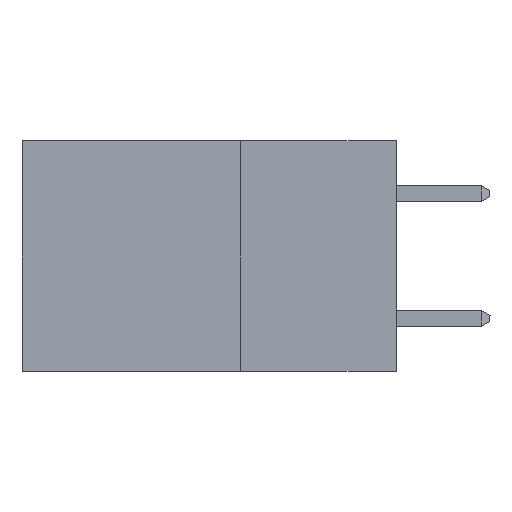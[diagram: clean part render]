
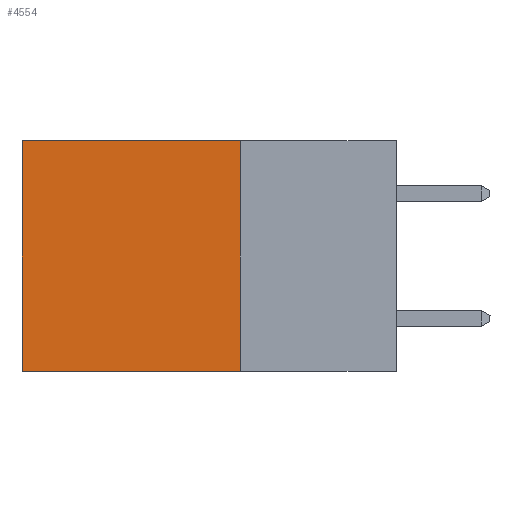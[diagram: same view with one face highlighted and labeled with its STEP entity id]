
A CAD part, left-side view. The second image highlights one B-rep face of the part: STEP entity #4554.
In plain terms, the highlighted planar face has unit normal (-1, 0, 0).
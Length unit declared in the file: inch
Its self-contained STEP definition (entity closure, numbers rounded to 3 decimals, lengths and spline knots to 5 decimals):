
#431 = EDGE_LOOP ( 'NONE', ( #10755, #3207, #16544, #15419 ) ) ;
#739 = CARTESIAN_POINT ( 'NONE',  ( 0.2615, 0.25, 0. ) ) ;
#2113 = EDGE_CURVE ( 'NONE', #11427, #13309, #3896, .T. ) ;
#2519 = LINE ( 'NONE', #15623, #10680 ) ;
#3207 = ORIENTED_EDGE ( 'NONE', *, *, #4720, .F. ) ;
#3378 = VECTOR ( 'NONE', #8932, 39.37008 ) ;
#3896 = LINE ( 'NONE', #9008, #3378 ) ;
#4066 = DIRECTION ( 'NONE',  ( 1., 0., 0. ) ) ;
#4404 = DIRECTION ( 'NONE',  ( 0., 1., 0. ) ) ;
#4472 = VERTEX_POINT ( 'NONE', #8683 ) ;
#4554 = ADVANCED_FACE ( 'NONE', ( #13385 ), #12192, .F. ) ;
#4720 = EDGE_CURVE ( 'NONE', #13309, #17518, #6117, .T. ) ;
#5331 = DIRECTION ( 'NONE',  ( 0., 0., -1. ) ) ;
#6117 = LINE ( 'NONE', #15782, #18546 ) ;
#6715 = LINE ( 'NONE', #16703, #10013 ) ;
#8683 = CARTESIAN_POINT ( 'NONE',  ( 0.2615, 0.6, 0. ) ) ;
#8932 = DIRECTION ( 'NONE',  ( 0., 0., -1. ) ) ;
#9008 = CARTESIAN_POINT ( 'NONE',  ( 0.2615, 0.25, -0.37 ) ) ;
#9054 = AXIS2_PLACEMENT_3D ( 'NONE', #13809, #4066, #15435 ) ;
#10013 = VECTOR ( 'NONE', #5331, 39.37008 ) ;
#10680 = VECTOR ( 'NONE', #14075, 39.37008 ) ;
#10755 = ORIENTED_EDGE ( 'NONE', *, *, #15216, .T. ) ;
#11427 = VERTEX_POINT ( 'NONE', #739 ) ;
#11560 = EDGE_CURVE ( 'NONE', #11427, #4472, #2519, .T. ) ;
#12192 = PLANE ( 'NONE',  #9054 ) ;
#13309 = VERTEX_POINT ( 'NONE', #17604 ) ;
#13385 = FACE_OUTER_BOUND ( 'NONE', #431, .T. ) ;
#13809 = CARTESIAN_POINT ( 'NONE',  ( 0.2615, 0.25, -0.37 ) ) ;
#14075 = DIRECTION ( 'NONE',  ( 0., 1., 0. ) ) ;
#15216 = EDGE_CURVE ( 'NONE', #4472, #17518, #6715, .T. ) ;
#15419 = ORIENTED_EDGE ( 'NONE', *, *, #11560, .T. ) ;
#15435 = DIRECTION ( 'NONE',  ( 0., 0., -1. ) ) ;
#15623 = CARTESIAN_POINT ( 'NONE',  ( 0.2615, 0.25, 0. ) ) ;
#15782 = CARTESIAN_POINT ( 'NONE',  ( 0.2615, 0.25, -0.37 ) ) ;
#16544 = ORIENTED_EDGE ( 'NONE', *, *, #2113, .F. ) ;
#16703 = CARTESIAN_POINT ( 'NONE',  ( 0.2615, 0.6, -0.37 ) ) ;
#17518 = VERTEX_POINT ( 'NONE', #19014 ) ;
#17604 = CARTESIAN_POINT ( 'NONE',  ( 0.2615, 0.25, -0.37 ) ) ;
#18546 = VECTOR ( 'NONE', #4404, 39.37008 ) ;
#19014 = CARTESIAN_POINT ( 'NONE',  ( 0.2615, 0.6, -0.37 ) ) ;
